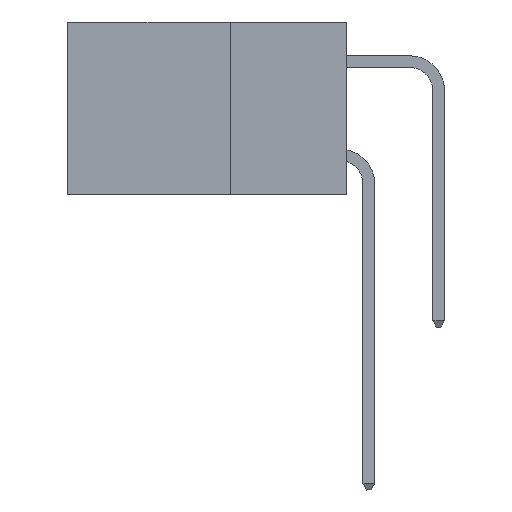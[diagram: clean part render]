
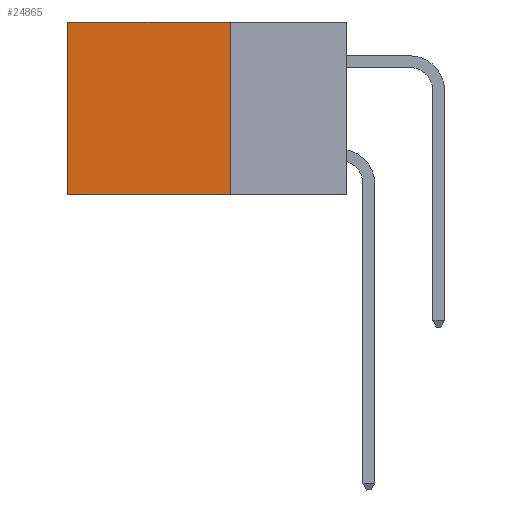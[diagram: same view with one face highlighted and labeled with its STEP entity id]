
A CAD part, left-side view. The second image highlights one B-rep face of the part: STEP entity #24865.
In plain terms, the highlighted planar face has unit normal (-1, 0, 0).
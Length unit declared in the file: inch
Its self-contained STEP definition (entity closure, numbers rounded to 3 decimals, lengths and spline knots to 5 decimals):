
#1166 = VECTOR ( 'NONE', #13985, 39.37008 ) ;
#1398 = ORIENTED_EDGE ( 'NONE', *, *, #23588, .T. ) ;
#2326 = FACE_OUTER_BOUND ( 'NONE', #8018, .T. ) ;
#2543 = VECTOR ( 'NONE', #5467, 39.37008 ) ;
#3398 = ORIENTED_EDGE ( 'NONE', *, *, #5359, .T. ) ;
#4070 = CARTESIAN_POINT ( 'NONE',  ( 0.2875, 0.25, 0. ) ) ;
#4875 = VERTEX_POINT ( 'NONE', #21975 ) ;
#5359 = EDGE_CURVE ( 'NONE', #4875, #24944, #11869, .T. ) ;
#5467 = DIRECTION ( 'NONE',  ( 0., 0., -1. ) ) ;
#6429 = CARTESIAN_POINT ( 'NONE',  ( 0.2875, 0.25, 0. ) ) ;
#6614 = ORIENTED_EDGE ( 'NONE', *, *, #14342, .F. ) ;
#7270 = VERTEX_POINT ( 'NONE', #24399 ) ;
#7865 = LINE ( 'NONE', #9283, #2543 ) ;
#8018 = EDGE_LOOP ( 'NONE', ( #1398, #20946, #6614, #3398 ) ) ;
#9038 = CARTESIAN_POINT ( 'NONE',  ( 0.2875, 0.25, -0.37 ) ) ;
#9283 = CARTESIAN_POINT ( 'NONE',  ( 0.2875, 0.6, 0. ) ) ;
#10172 = LINE ( 'NONE', #6429, #1166 ) ;
#10376 = PLANE ( 'NONE',  #16545 ) ;
#11767 = CARTESIAN_POINT ( 'NONE',  ( 0.2875, 0.25, -0.37 ) ) ;
#11869 = LINE ( 'NONE', #4070, #18335 ) ;
#13985 = DIRECTION ( 'NONE',  ( 0., 0., -1. ) ) ;
#14342 = EDGE_CURVE ( 'NONE', #4875, #20969, #10172, .T. ) ;
#16545 = AXIS2_PLACEMENT_3D ( 'NONE', #24724, #22026, #16870 ) ;
#16779 = EDGE_CURVE ( 'NONE', #20969, #7270, #20464, .T. ) ;
#16870 = DIRECTION ( 'NONE',  ( 0., 0., -1. ) ) ;
#18335 = VECTOR ( 'NONE', #20622, 39.37008 ) ;
#20464 = LINE ( 'NONE', #11767, #21974 ) ;
#20622 = DIRECTION ( 'NONE',  ( 0., 1., 0. ) ) ;
#20946 = ORIENTED_EDGE ( 'NONE', *, *, #16779, .F. ) ;
#20969 = VERTEX_POINT ( 'NONE', #9038 ) ;
#21974 = VECTOR ( 'NONE', #25385, 39.37008 ) ;
#21975 = CARTESIAN_POINT ( 'NONE',  ( 0.2875, 0.25, 0. ) ) ;
#22026 = DIRECTION ( 'NONE',  ( 1., 0., 0. ) ) ;
#22191 = CARTESIAN_POINT ( 'NONE',  ( 0.2875, 0.6, 0. ) ) ;
#23588 = EDGE_CURVE ( 'NONE', #24944, #7270, #7865, .T. ) ;
#24399 = CARTESIAN_POINT ( 'NONE',  ( 0.2875, 0.6, -0.37 ) ) ;
#24724 = CARTESIAN_POINT ( 'NONE',  ( 0.2875, 0.25, 0. ) ) ;
#24865 = ADVANCED_FACE ( 'NONE', ( #2326 ), #10376, .F. ) ;
#24944 = VERTEX_POINT ( 'NONE', #22191 ) ;
#25385 = DIRECTION ( 'NONE',  ( 0., 1., 0. ) ) ;
